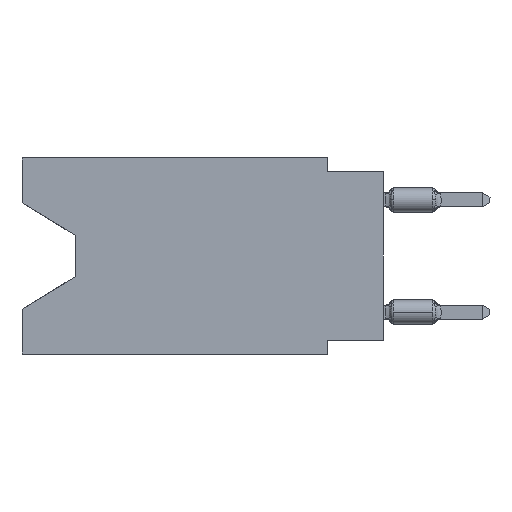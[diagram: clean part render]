
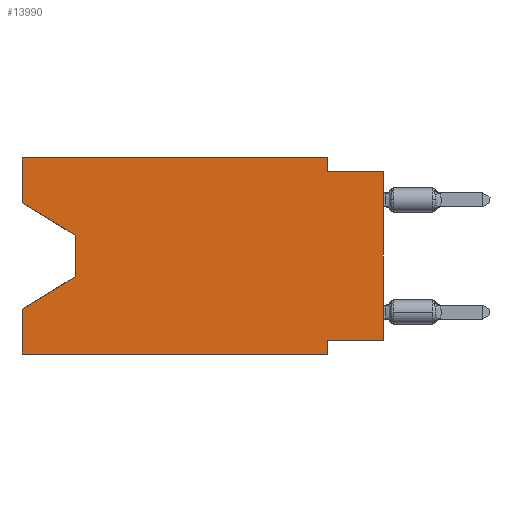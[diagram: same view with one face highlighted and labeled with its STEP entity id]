
A CAD part, left-side view. The second image highlights one B-rep face of the part: STEP entity #13990.
In plain terms, the highlighted planar face has unit normal (-1, 0, 0).
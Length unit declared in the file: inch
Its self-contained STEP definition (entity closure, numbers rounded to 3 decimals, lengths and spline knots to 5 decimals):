
#298 = ORIENTED_EDGE ( 'NONE', *, *, #34199, .T. ) ;
#361 = VERTEX_POINT ( 'NONE', #1147 ) ;
#386 = EDGE_CURVE ( 'NONE', #39965, #25491, #32989, .T. ) ;
#457 = LINE ( 'NONE', #28294, #41420 ) ;
#500 = DIRECTION ( 'NONE',  ( 0., 0., -1. ) ) ;
#868 = DIRECTION ( 'NONE',  ( 0., 0., 1. ) ) ;
#987 = EDGE_CURVE ( 'NONE', #14937, #30361, #28253, .T. ) ;
#1147 = CARTESIAN_POINT ( 'NONE',  ( 0., 0.1, -0.35 ) ) ;
#1359 = ORIENTED_EDGE ( 'NONE', *, *, #987, .F. ) ;
#1632 = CARTESIAN_POINT ( 'NONE',  ( 0., 0., -0.025 ) ) ;
#3468 = VECTOR ( 'NONE', #29704, 39.37008 ) ;
#3561 = ORIENTED_EDGE ( 'NONE', *, *, #37363, .F. ) ;
#3730 = DIRECTION ( 'NONE',  ( 0., 0., -1. ) ) ;
#3924 = DIRECTION ( 'NONE',  ( 0., 1., 0. ) ) ;
#3992 = ORIENTED_EDGE ( 'NONE', *, *, #386, .F. ) ;
#4384 = CARTESIAN_POINT ( 'NONE',  ( 0., 0.1, -0.325 ) ) ;
#4548 = CARTESIAN_POINT ( 'NONE',  ( 0., 0.1, -0.35 ) ) ;
#4758 = EDGE_CURVE ( 'NONE', #8359, #12434, #26461, .T. ) ;
#4967 = CARTESIAN_POINT ( 'NONE',  ( 0., 0.55, -0.212 ) ) ;
#5557 = ORIENTED_EDGE ( 'NONE', *, *, #5995, .F. ) ;
#5995 = EDGE_CURVE ( 'NONE', #33979, #46157, #35893, .T. ) ;
#6876 = DIRECTION ( 'NONE',  ( 0., 0., 1. ) ) ;
#7200 = LINE ( 'NONE', #35751, #41539 ) ;
#7803 = CARTESIAN_POINT ( 'NONE',  ( 0., 0.645, -0.35 ) ) ;
#8238 = EDGE_CURVE ( 'NONE', #30361, #361, #24872, .T. ) ;
#8359 = VERTEX_POINT ( 'NONE', #16210 ) ;
#8453 = VECTOR ( 'NONE', #22063, 39.37008 ) ;
#8950 = CARTESIAN_POINT ( 'NONE',  ( 0., 0.645, 0. ) ) ;
#10395 = LINE ( 'NONE', #38744, #18411 ) ;
#11036 = EDGE_CURVE ( 'NONE', #43681, #39965, #27256, .T. ) ;
#11464 = ORIENTED_EDGE ( 'NONE', *, *, #8238, .F. ) ;
#11541 = DIRECTION ( 'NONE',  ( 0., 0., -1. ) ) ;
#12117 = EDGE_CURVE ( 'NONE', #16433, #361, #39649, .T. ) ;
#12434 = VERTEX_POINT ( 'NONE', #25319 ) ;
#13087 = ORIENTED_EDGE ( 'NONE', *, *, #28260, .T. ) ;
#13990 = ADVANCED_FACE ( 'NONE', ( #25297 ), #32565, .F. ) ;
#14595 = VECTOR ( 'NONE', #11541, 39.37008 ) ;
#14937 = VERTEX_POINT ( 'NONE', #29824 ) ;
#16097 = VECTOR ( 'NONE', #19234, 39.37008 ) ;
#16210 = CARTESIAN_POINT ( 'NONE',  ( 0., 0.55, -0.212 ) ) ;
#16433 = VERTEX_POINT ( 'NONE', #34929 ) ;
#16496 = DIRECTION ( 'NONE',  ( 0., -0.855, -0.519 ) ) ;
#17045 = ORIENTED_EDGE ( 'NONE', *, *, #4758, .T. ) ;
#18237 = CARTESIAN_POINT ( 'NONE',  ( 0., 0.645, 0. ) ) ;
#18411 = VECTOR ( 'NONE', #16496, 39.37008 ) ;
#18991 = CARTESIAN_POINT ( 'NONE',  ( 0., 0.645, 0. ) ) ;
#19234 = DIRECTION ( 'NONE',  ( 0., 0.855, -0.519 ) ) ;
#20025 = CARTESIAN_POINT ( 'NONE',  ( 0., 0.645, 0. ) ) ;
#20461 = CARTESIAN_POINT ( 'NONE',  ( 0., 0.1, 0. ) ) ;
#21951 = VERTEX_POINT ( 'NONE', #41713 ) ;
#22063 = DIRECTION ( 'NONE',  ( 0., -1., 0. ) ) ;
#24872 = LINE ( 'NONE', #4548, #14595 ) ;
#25297 = FACE_OUTER_BOUND ( 'NONE', #44575, .T. ) ;
#25319 = CARTESIAN_POINT ( 'NONE',  ( 0., 0.645, -0.26975 ) ) ;
#25491 = VERTEX_POINT ( 'NONE', #20461 ) ;
#26461 = LINE ( 'NONE', #4967, #16097 ) ;
#27256 = LINE ( 'NONE', #20025, #28623 ) ;
#27492 = DIRECTION ( 'NONE',  ( 0., 0., 1. ) ) ;
#28253 = LINE ( 'NONE', #39289, #35551 ) ;
#28260 = EDGE_CURVE ( 'NONE', #21951, #8359, #33805, .T. ) ;
#28294 = CARTESIAN_POINT ( 'NONE',  ( 0., 0.1, 0. ) ) ;
#28623 = VECTOR ( 'NONE', #27492, 39.37008 ) ;
#28709 = CARTESIAN_POINT ( 'NONE',  ( 0., 0.1, -0.025 ) ) ;
#29704 = DIRECTION ( 'NONE',  ( 0., -1., 0. ) ) ;
#29824 = CARTESIAN_POINT ( 'NONE',  ( 0., 0., -0.325 ) ) ;
#29843 = DIRECTION ( 'NONE',  ( 0., 0., -1. ) ) ;
#29940 = ORIENTED_EDGE ( 'NONE', *, *, #33956, .F. ) ;
#30361 = VERTEX_POINT ( 'NONE', #4384 ) ;
#30652 = EDGE_CURVE ( 'NONE', #14937, #46157, #42018, .T. ) ;
#30692 = CARTESIAN_POINT ( 'NONE',  ( 0., 0., -0.025 ) ) ;
#32565 = PLANE ( 'NONE',  #44472 ) ;
#32989 = LINE ( 'NONE', #18237, #3468 ) ;
#33495 = DIRECTION ( 'NONE',  ( 0., -1., 0. ) ) ;
#33805 = LINE ( 'NONE', #34026, #38284 ) ;
#33956 = EDGE_CURVE ( 'NONE', #16433, #12434, #7200, .T. ) ;
#33979 = VERTEX_POINT ( 'NONE', #28709 ) ;
#34026 = CARTESIAN_POINT ( 'NONE',  ( 0., 0.55, -0.138 ) ) ;
#34199 = EDGE_CURVE ( 'NONE', #43681, #21951, #10395, .T. ) ;
#34929 = CARTESIAN_POINT ( 'NONE',  ( 0., 0.645, -0.35 ) ) ;
#35551 = VECTOR ( 'NONE', #3924, 39.37008 ) ;
#35751 = CARTESIAN_POINT ( 'NONE',  ( 0., 0.645, 0. ) ) ;
#35893 = LINE ( 'NONE', #1632, #39285 ) ;
#36978 = ORIENTED_EDGE ( 'NONE', *, *, #11036, .F. ) ;
#37236 = ORIENTED_EDGE ( 'NONE', *, *, #30652, .T. ) ;
#37363 = EDGE_CURVE ( 'NONE', #25491, #33979, #457, .T. ) ;
#38257 = CARTESIAN_POINT ( 'NONE',  ( 0., 0., 0. ) ) ;
#38284 = VECTOR ( 'NONE', #29843, 39.37008 ) ;
#38744 = CARTESIAN_POINT ( 'NONE',  ( 0., 0.645, -0.08025 ) ) ;
#39285 = VECTOR ( 'NONE', #33495, 39.37008 ) ;
#39289 = CARTESIAN_POINT ( 'NONE',  ( 0., 0., -0.325 ) ) ;
#39649 = LINE ( 'NONE', #7803, #8453 ) ;
#39965 = VERTEX_POINT ( 'NONE', #8950 ) ;
#40327 = DIRECTION ( 'NONE',  ( 1., 0., 0. ) ) ;
#41420 = VECTOR ( 'NONE', #3730, 39.37008 ) ;
#41539 = VECTOR ( 'NONE', #868, 39.37008 ) ;
#41713 = CARTESIAN_POINT ( 'NONE',  ( 0., 0.55, -0.138 ) ) ;
#42018 = LINE ( 'NONE', #38257, #45968 ) ;
#43681 = VERTEX_POINT ( 'NONE', #45959 ) ;
#44472 = AXIS2_PLACEMENT_3D ( 'NONE', #18991, #40327, #500 ) ;
#44575 = EDGE_LOOP ( 'NONE', ( #298, #13087, #17045, #29940, #44823, #11464, #1359, #37236, #5557, #3561, #3992, #36978 ) ) ;
#44823 = ORIENTED_EDGE ( 'NONE', *, *, #12117, .T. ) ;
#45959 = CARTESIAN_POINT ( 'NONE',  ( 0., 0.645, -0.08025 ) ) ;
#45968 = VECTOR ( 'NONE', #6876, 39.37008 ) ;
#46157 = VERTEX_POINT ( 'NONE', #30692 ) ;
